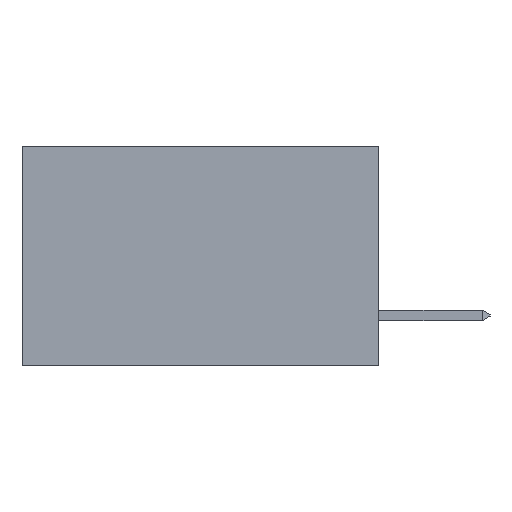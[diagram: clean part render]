
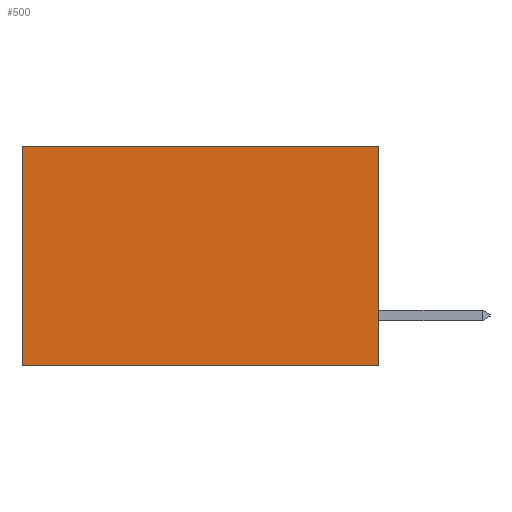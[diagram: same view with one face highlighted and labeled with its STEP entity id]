
A CAD part, left-side view. The second image highlights one B-rep face of the part: STEP entity #500.
In plain terms, the highlighted planar face has unit normal (-1, 0, 0).
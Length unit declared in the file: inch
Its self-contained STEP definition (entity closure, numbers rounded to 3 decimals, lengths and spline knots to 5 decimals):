
#146 = CARTESIAN_POINT ( 'NONE',  ( 0.2615, 0., -0.37 ) ) ;
#321 = LINE ( 'NONE', #1607, #6109 ) ;
#500 = ADVANCED_FACE ( 'NONE', ( #8015 ), #7285, .F. ) ;
#760 = EDGE_CURVE ( 'NONE', #2866, #7195, #8539, .T. ) ;
#926 = VECTOR ( 'NONE', #13924, 39.37008 ) ;
#1134 = CARTESIAN_POINT ( 'NONE',  ( 0.2615, 0., 0. ) ) ;
#1151 = CARTESIAN_POINT ( 'NONE',  ( 0.2615, 0.6, -0.37 ) ) ;
#1607 = CARTESIAN_POINT ( 'NONE',  ( 0.2615, 0.6, -0.37 ) ) ;
#1611 = LINE ( 'NONE', #5168, #926 ) ;
#2138 = LINE ( 'NONE', #146, #10564 ) ;
#2866 = VERTEX_POINT ( 'NONE', #7682 ) ;
#4000 = DIRECTION ( 'NONE',  ( 0., 0., -1. ) ) ;
#4209 = CARTESIAN_POINT ( 'NONE',  ( 0.2615, 0., -0.37 ) ) ;
#4439 = VECTOR ( 'NONE', #5500, 39.37008 ) ;
#5168 = CARTESIAN_POINT ( 'NONE',  ( 0.2615, 0., 0. ) ) ;
#5500 = DIRECTION ( 'NONE',  ( 0., 1., 0. ) ) ;
#6109 = VECTOR ( 'NONE', #4000, 39.37008 ) ;
#6150 = EDGE_CURVE ( 'NONE', #9058, #7195, #321, .T. ) ;
#6217 = AXIS2_PLACEMENT_3D ( 'NONE', #14412, #8598, #8014 ) ;
#6997 = EDGE_LOOP ( 'NONE', ( #8304, #10604, #11429, #11243 ) ) ;
#7195 = VERTEX_POINT ( 'NONE', #1151 ) ;
#7285 = PLANE ( 'NONE',  #6217 ) ;
#7682 = CARTESIAN_POINT ( 'NONE',  ( 0.2615, 0., -0.37 ) ) ;
#7844 = VERTEX_POINT ( 'NONE', #1134 ) ;
#8014 = DIRECTION ( 'NONE',  ( 0., 0., -1. ) ) ;
#8015 = FACE_OUTER_BOUND ( 'NONE', #6997, .T. ) ;
#8304 = ORIENTED_EDGE ( 'NONE', *, *, #6150, .T. ) ;
#8539 = LINE ( 'NONE', #4209, #4439 ) ;
#8598 = DIRECTION ( 'NONE',  ( 1., 0., 0. ) ) ;
#8756 = EDGE_CURVE ( 'NONE', #7844, #2866, #2138, .T. ) ;
#9058 = VERTEX_POINT ( 'NONE', #9824 ) ;
#9824 = CARTESIAN_POINT ( 'NONE',  ( 0.2615, 0.6, 0. ) ) ;
#10433 = DIRECTION ( 'NONE',  ( 0., 0., -1. ) ) ;
#10564 = VECTOR ( 'NONE', #10433, 39.37008 ) ;
#10604 = ORIENTED_EDGE ( 'NONE', *, *, #760, .F. ) ;
#11243 = ORIENTED_EDGE ( 'NONE', *, *, #13438, .T. ) ;
#11429 = ORIENTED_EDGE ( 'NONE', *, *, #8756, .F. ) ;
#13438 = EDGE_CURVE ( 'NONE', #7844, #9058, #1611, .T. ) ;
#13924 = DIRECTION ( 'NONE',  ( 0., 1., 0. ) ) ;
#14412 = CARTESIAN_POINT ( 'NONE',  ( 0.2615, 0., -0.37 ) ) ;
